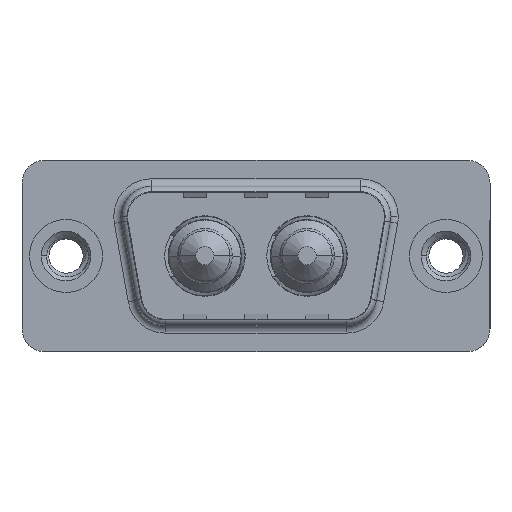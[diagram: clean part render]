
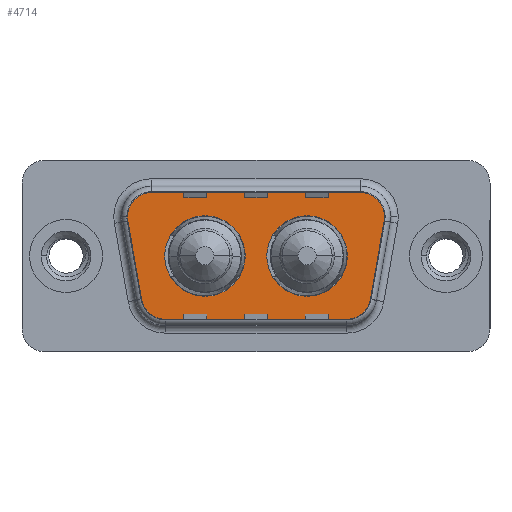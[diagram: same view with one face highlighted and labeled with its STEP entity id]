
A CAD part, top view. The second image highlights one B-rep face of the part: STEP entity #4714.
In plain terms, the highlighted planar face has unit normal (0, 0, 1).
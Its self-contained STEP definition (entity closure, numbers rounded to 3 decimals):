
#78 = AXIS2_PLACEMENT_3D ( 'NONE', #7810, #8225, #2524 ) ;
#90 = VERTEX_POINT ( 'NONE', #392 ) ;
#392 = CARTESIAN_POINT ( 'NONE',  ( 11.79, 0., 0. ) ) ;
#508 = EDGE_CURVE ( 'NONE', #4862, #9108, #6476, .T. ) ;
#560 = CIRCLE ( 'NONE', #10920, 2. ) ;
#689 = DIRECTION ( 'NONE',  ( 0., 0., 1. ) ) ;
#786 = VERTEX_POINT ( 'NONE', #4329 ) ;
#797 = CARTESIAN_POINT ( 'NONE',  ( 6.459, -4.9, 0. ) ) ;
#826 = VECTOR ( 'NONE', #9226, 1000. ) ;
#956 = CIRCLE ( 'NONE', #4603, 2. ) ;
#1107 = CARTESIAN_POINT ( 'NONE',  ( 5.436, 4.9, 0. ) ) ;
#1168 = ORIENTED_EDGE ( 'NONE', *, *, #1904, .T. ) ;
#1530 = CARTESIAN_POINT ( 'NONE',  ( 6.459, -2.9, 0. ) ) ;
#1676 = DIRECTION ( 'NONE',  ( 1., 0., 0. ) ) ;
#1678 = CARTESIAN_POINT ( 'NONE',  ( 15.86, 0., 0. ) ) ;
#1755 = CIRCLE ( 'NONE', #78, 2.65 ) ;
#1890 = VECTOR ( 'NONE', #3857, 1000. ) ;
#1902 = CARTESIAN_POINT ( 'NONE',  ( 9.14, 0., 0. ) ) ;
#1904 = EDGE_CURVE ( 'NONE', #7876, #9760, #5192, .T. ) ;
#1926 = ORIENTED_EDGE ( 'NONE', *, *, #10321, .T. ) ;
#1978 = DIRECTION ( 'NONE',  ( 0., 0., 1. ) ) ;
#1980 = FACE_BOUND ( 'NONE', #8606, .T. ) ;
#2080 = CARTESIAN_POINT ( 'NONE',  ( 21.564, 2.9, 0. ) ) ;
#2116 = EDGE_CURVE ( 'NONE', #10262, #6750, #10381, .T. ) ;
#2148 = CIRCLE ( 'NONE', #2418, 2.65 ) ;
#2223 = EDGE_CURVE ( 'NONE', #90, #8964, #2148, .T. ) ;
#2315 = EDGE_CURVE ( 'NONE', #6750, #7876, #10244, .T. ) ;
#2368 = VERTEX_POINT ( 'NONE', #2080 ) ;
#2371 = CARTESIAN_POINT ( 'NONE',  ( 19.564, 2.9, 0. ) ) ;
#2418 = AXIS2_PLACEMENT_3D ( 'NONE', #3389, #8760, #9560 ) ;
#2506 = DIRECTION ( 'NONE',  ( 0., 0., 1. ) ) ;
#2524 = DIRECTION ( 'NONE',  ( 1., 0., 0. ) ) ;
#2580 = AXIS2_PLACEMENT_3D ( 'NONE', #1902, #8062, #2756 ) ;
#2581 = EDGE_CURVE ( 'NONE', #2368, #786, #956, .T. ) ;
#2667 = AXIS2_PLACEMENT_3D ( 'NONE', #7239, #1978, #8149 ) ;
#2756 = DIRECTION ( 'NONE',  ( 1., 0., 0. ) ) ;
#2789 = AXIS2_PLACEMENT_3D ( 'NONE', #5009, #5849, #1676 ) ;
#2848 = CARTESIAN_POINT ( 'NONE',  ( 21.534, 2.553, 0. ) ) ;
#2853 = EDGE_CURVE ( 'NONE', #6108, #8550, #10234, .T. ) ;
#2982 = EDGE_CURVE ( 'NONE', #8550, #6108, #1755, .T. ) ;
#3125 = ORIENTED_EDGE ( 'NONE', *, *, #2853, .F. ) ;
#3190 = ORIENTED_EDGE ( 'NONE', *, *, #508, .T. ) ;
#3279 = DIRECTION ( 'NONE',  ( -1., 0., 0. ) ) ;
#3389 = CARTESIAN_POINT ( 'NONE',  ( 9.14, 0., 0. ) ) ;
#3475 = CARTESIAN_POINT ( 'NONE',  ( 18.541, -4.9, 0. ) ) ;
#3608 = DIRECTION ( 'NONE',  ( 0.174, -0.985, 0. ) ) ;
#3786 = ORIENTED_EDGE ( 'NONE', *, *, #2315, .T. ) ;
#3855 = ORIENTED_EDGE ( 'NONE', *, *, #10020, .T. ) ;
#3857 = DIRECTION ( 'NONE',  ( -1., 0., 0. ) ) ;
#3938 = CARTESIAN_POINT ( 'NONE',  ( 3.466, 2.553, 0. ) ) ;
#3955 = CARTESIAN_POINT ( 'NONE',  ( 3.466, 2.553, 0. ) ) ;
#3981 = CARTESIAN_POINT ( 'NONE',  ( 4.489, -3.247, 0. ) ) ;
#3989 = CARTESIAN_POINT ( 'NONE',  ( 20.511, -3.247, 0. ) ) ;
#4050 = ORIENTED_EDGE ( 'NONE', *, *, #9620, .T. ) ;
#4124 = DIRECTION ( 'NONE',  ( -1., 0., 0. ) ) ;
#4132 = ORIENTED_EDGE ( 'NONE', *, *, #2223, .F. ) ;
#4209 = LINE ( 'NONE', #10113, #1890 ) ;
#4220 = AXIS2_PLACEMENT_3D ( 'NONE', #1530, #689, #4124 ) ;
#4329 = CARTESIAN_POINT ( 'NONE',  ( 19.564, 4.9, 0. ) ) ;
#4365 = CARTESIAN_POINT ( 'NONE',  ( 6.459, -4.9, 0. ) ) ;
#4377 = AXIS2_PLACEMENT_3D ( 'NONE', #1678, #5582, #8791 ) ;
#4509 = CARTESIAN_POINT ( 'NONE',  ( 18.51, 0., 0. ) ) ;
#4558 = ORIENTED_EDGE ( 'NONE', *, *, #2581, .T. ) ;
#4603 = AXIS2_PLACEMENT_3D ( 'NONE', #6039, #6700, #10345 ) ;
#4714 = ADVANCED_FACE ( 'NONE', ( #11477, #1980, #11198 ), #5572, .T. ) ;
#4862 = VERTEX_POINT ( 'NONE', #3989 ) ;
#5009 = CARTESIAN_POINT ( 'NONE',  ( 18.541, -2.9, 0. ) ) ;
#5192 = LINE ( 'NONE', #797, #826 ) ;
#5319 = ORIENTED_EDGE ( 'NONE', *, *, #2982, .F. ) ;
#5572 = PLANE ( 'NONE',  #2789 ) ;
#5582 = DIRECTION ( 'NONE',  ( 0., 0., 1. ) ) ;
#5849 = DIRECTION ( 'NONE',  ( 0., 0., 1. ) ) ;
#5863 = CARTESIAN_POINT ( 'NONE',  ( 6.49, 0., 0. ) ) ;
#5936 = EDGE_LOOP ( 'NONE', ( #5319, #3125 ) ) ;
#6021 = CARTESIAN_POINT ( 'NONE',  ( 21.534, 2.553, 0. ) ) ;
#6039 = CARTESIAN_POINT ( 'NONE',  ( 19.564, 2.9, 0. ) ) ;
#6108 = VERTEX_POINT ( 'NONE', #11128 ) ;
#6476 = LINE ( 'NONE', #2848, #8575 ) ;
#6700 = DIRECTION ( 'NONE',  ( 0., 0., 1. ) ) ;
#6750 = VERTEX_POINT ( 'NONE', #3981 ) ;
#7187 = AXIS2_PLACEMENT_3D ( 'NONE', #7809, #2506, #8737 ) ;
#7239 = CARTESIAN_POINT ( 'NONE',  ( 5.436, 2.9, 0. ) ) ;
#7809 = CARTESIAN_POINT ( 'NONE',  ( 18.541, -2.9, 0. ) ) ;
#7810 = CARTESIAN_POINT ( 'NONE',  ( 15.86, 0., 0. ) ) ;
#7876 = VERTEX_POINT ( 'NONE', #4365 ) ;
#7972 = ORIENTED_EDGE ( 'NONE', *, *, #2116, .T. ) ;
#8062 = DIRECTION ( 'NONE',  ( 0., 0., 1. ) ) ;
#8149 = DIRECTION ( 'NONE',  ( 1., 0., 0. ) ) ;
#8225 = DIRECTION ( 'NONE',  ( 0., 0., 1. ) ) ;
#8526 = CIRCLE ( 'NONE', #7187, 2. ) ;
#8542 = EDGE_CURVE ( 'NONE', #8964, #90, #8570, .T. ) ;
#8550 = VERTEX_POINT ( 'NONE', #4509 ) ;
#8570 = CIRCLE ( 'NONE', #2580, 2.65 ) ;
#8575 = VECTOR ( 'NONE', #9438, 1000. ) ;
#8599 = DIRECTION ( 'NONE',  ( 0., 0., 1. ) ) ;
#8606 = EDGE_LOOP ( 'NONE', ( #4132, #9146 ) ) ;
#8737 = DIRECTION ( 'NONE',  ( 1., 0., 0. ) ) ;
#8760 = DIRECTION ( 'NONE',  ( 0., 0., 1. ) ) ;
#8791 = DIRECTION ( 'NONE',  ( 1., 0., 0. ) ) ;
#8835 = VECTOR ( 'NONE', #3608, 1000. ) ;
#8878 = EDGE_LOOP ( 'NONE', ( #1926, #3190, #4050, #4558, #10337, #3855, #7972, #3786, #1168 ) ) ;
#8964 = VERTEX_POINT ( 'NONE', #5863 ) ;
#9108 = VERTEX_POINT ( 'NONE', #6021 ) ;
#9146 = ORIENTED_EDGE ( 'NONE', *, *, #8542, .F. ) ;
#9226 = DIRECTION ( 'NONE',  ( 1., 0., 0. ) ) ;
#9438 = DIRECTION ( 'NONE',  ( 0.174, 0.985, 0. ) ) ;
#9560 = DIRECTION ( 'NONE',  ( 1., 0., 0. ) ) ;
#9620 = EDGE_CURVE ( 'NONE', #9108, #2368, #560, .T. ) ;
#9760 = VERTEX_POINT ( 'NONE', #3475 ) ;
#10020 = EDGE_CURVE ( 'NONE', #10588, #10262, #11396, .T. ) ;
#10113 = CARTESIAN_POINT ( 'NONE',  ( 5.436, 4.9, 0. ) ) ;
#10234 = CIRCLE ( 'NONE', #4377, 2.65 ) ;
#10244 = CIRCLE ( 'NONE', #4220, 2. ) ;
#10262 = VERTEX_POINT ( 'NONE', #3938 ) ;
#10321 = EDGE_CURVE ( 'NONE', #9760, #4862, #8526, .T. ) ;
#10337 = ORIENTED_EDGE ( 'NONE', *, *, #11202, .T. ) ;
#10345 = DIRECTION ( 'NONE',  ( -1., 0., 0. ) ) ;
#10381 = LINE ( 'NONE', #3955, #8835 ) ;
#10588 = VERTEX_POINT ( 'NONE', #1107 ) ;
#10920 = AXIS2_PLACEMENT_3D ( 'NONE', #2371, #8599, #3279 ) ;
#11128 = CARTESIAN_POINT ( 'NONE',  ( 13.21, 0., 0. ) ) ;
#11198 = FACE_OUTER_BOUND ( 'NONE', #8878, .T. ) ;
#11202 = EDGE_CURVE ( 'NONE', #786, #10588, #4209, .T. ) ;
#11396 = CIRCLE ( 'NONE', #2667, 2. ) ;
#11477 = FACE_BOUND ( 'NONE', #5936, .T. ) ;
